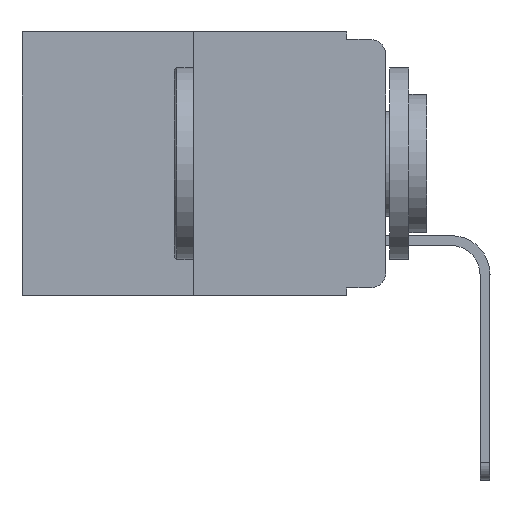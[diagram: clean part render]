
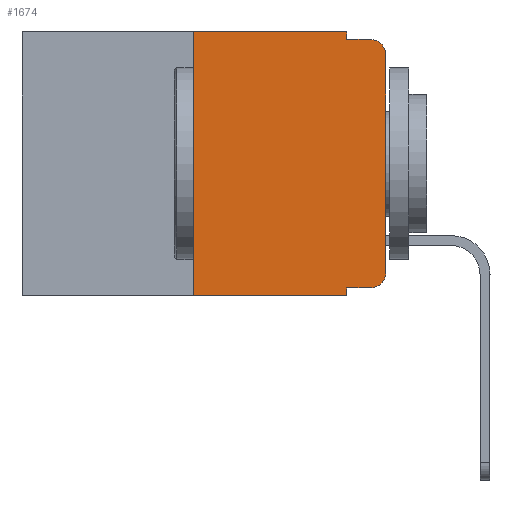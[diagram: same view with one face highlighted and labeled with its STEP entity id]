
A CAD part, left-side view. The second image highlights one B-rep face of the part: STEP entity #1674.
In plain terms, the highlighted planar face has unit normal (-1, 0, 0).
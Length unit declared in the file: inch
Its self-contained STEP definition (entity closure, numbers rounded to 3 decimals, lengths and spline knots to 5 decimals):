
#30 = LINE ( 'NONE', #6176, #9554 ) ;
#115 = VERTEX_POINT ( 'NONE', #6775 ) ;
#348 = DIRECTION ( 'NONE',  ( 0., 0., -1. ) ) ;
#703 = DIRECTION ( 'NONE',  ( 1., 0., 0. ) ) ;
#757 = VECTOR ( 'NONE', #9852, 39.37008 ) ;
#905 = EDGE_CURVE ( 'NONE', #6582, #11496, #3817, .T. ) ;
#1418 = LINE ( 'NONE', #9605, #4069 ) ;
#1454 = CARTESIAN_POINT ( 'NONE',  ( 0., 0., 0. ) ) ;
#1549 = ORIENTED_EDGE ( 'NONE', *, *, #5452, .T. ) ;
#1674 = ADVANCED_FACE ( 'NONE', ( #9595 ), #4246, .F. ) ;
#1706 = DIRECTION ( 'NONE',  ( 0., 0., 1. ) ) ;
#1743 = CARTESIAN_POINT ( 'NONE',  ( 0., 0.25, 0. ) ) ;
#1867 = VECTOR ( 'NONE', #6703, 39.37008 ) ;
#1996 = ORIENTED_EDGE ( 'NONE', *, *, #905, .F. ) ;
#2010 = CIRCLE ( 'NONE', #9799, 0.02 ) ;
#2052 = CARTESIAN_POINT ( 'NONE',  ( 0., 0.02, -0.313 ) ) ;
#2096 = LINE ( 'NONE', #9301, #5135 ) ;
#2180 = CARTESIAN_POINT ( 'NONE',  ( 0., 0.051, -0.01 ) ) ;
#2213 = DIRECTION ( 'NONE',  ( 0., -1., 0. ) ) ;
#2321 = ORIENTED_EDGE ( 'NONE', *, *, #10936, .T. ) ;
#2411 = VERTEX_POINT ( 'NONE', #9556 ) ;
#2516 = CARTESIAN_POINT ( 'NONE',  ( 0., 0.051, 0. ) ) ;
#2579 = AXIS2_PLACEMENT_3D ( 'NONE', #10174, #8378, #4041 ) ;
#2709 = DIRECTION ( 'NONE',  ( 0., -1., 0. ) ) ;
#2853 = VECTOR ( 'NONE', #9099, 39.37008 ) ;
#2990 = CARTESIAN_POINT ( 'NONE',  ( 0., 0.02, -0.333 ) ) ;
#3325 = ORIENTED_EDGE ( 'NONE', *, *, #10049, .T. ) ;
#3437 = CARTESIAN_POINT ( 'NONE',  ( 0., 0., -0.313 ) ) ;
#3559 = LINE ( 'NONE', #3613, #757 ) ;
#3613 = CARTESIAN_POINT ( 'NONE',  ( 0., 0.051, 0. ) ) ;
#3817 = LINE ( 'NONE', #5530, #2853 ) ;
#3937 = VECTOR ( 'NONE', #2709, 39.37008 ) ;
#4041 = DIRECTION ( 'NONE',  ( 0., 0., -1. ) ) ;
#4069 = VECTOR ( 'NONE', #5091, 39.37008 ) ;
#4124 = ORIENTED_EDGE ( 'NONE', *, *, #9107, .F. ) ;
#4174 = CARTESIAN_POINT ( 'NONE',  ( 0., 0.25, -0.343 ) ) ;
#4246 = PLANE ( 'NONE',  #5013 ) ;
#4949 = VERTEX_POINT ( 'NONE', #9428 ) ;
#5013 = AXIS2_PLACEMENT_3D ( 'NONE', #5121, #703, #6805 ) ;
#5091 = DIRECTION ( 'NONE',  ( 0., -1., 0. ) ) ;
#5121 = CARTESIAN_POINT ( 'NONE',  ( 0., 0.473, 0. ) ) ;
#5135 = VECTOR ( 'NONE', #2213, 39.37008 ) ;
#5156 = ORIENTED_EDGE ( 'NONE', *, *, #6040, .F. ) ;
#5393 = ORIENTED_EDGE ( 'NONE', *, *, #9227, .T. ) ;
#5452 = EDGE_CURVE ( 'NONE', #7818, #2411, #2096, .T. ) ;
#5530 = CARTESIAN_POINT ( 'NONE',  ( 0., 0.051, 0. ) ) ;
#5874 = VECTOR ( 'NONE', #1706, 39.37008 ) ;
#6040 = EDGE_CURVE ( 'NONE', #11496, #8912, #30, .T. ) ;
#6176 = CARTESIAN_POINT ( 'NONE',  ( 0., 0.051, -0.01 ) ) ;
#6582 = VERTEX_POINT ( 'NONE', #2516 ) ;
#6680 = LINE ( 'NONE', #9794, #3937 ) ;
#6703 = DIRECTION ( 'NONE',  ( 0., 0., 1. ) ) ;
#6775 = CARTESIAN_POINT ( 'NONE',  ( 0., 0.051, -0.333 ) ) ;
#6805 = DIRECTION ( 'NONE',  ( 0., 0., -1. ) ) ;
#7450 = DIRECTION ( 'NONE',  ( -1., 0., 0. ) ) ;
#7818 = VERTEX_POINT ( 'NONE', #4174 ) ;
#8344 = LINE ( 'NONE', #1743, #5874 ) ;
#8378 = DIRECTION ( 'NONE',  ( -1., 0., 0. ) ) ;
#8449 = CARTESIAN_POINT ( 'NONE',  ( 0., 0.02, -0.01 ) ) ;
#8583 = EDGE_LOOP ( 'NONE', ( #9252, #2321, #5156, #1996, #9936, #9468, #1549, #4124, #3325, #5393 ) ) ;
#8822 = DIRECTION ( 'NONE',  ( 0., -1., 0. ) ) ;
#8912 = VERTEX_POINT ( 'NONE', #8449 ) ;
#9099 = DIRECTION ( 'NONE',  ( 0., 0., -1. ) ) ;
#9107 = EDGE_CURVE ( 'NONE', #115, #2411, #3559, .T. ) ;
#9227 = EDGE_CURVE ( 'NONE', #9239, #11197, #2010, .T. ) ;
#9239 = VERTEX_POINT ( 'NONE', #2990 ) ;
#9252 = ORIENTED_EDGE ( 'NONE', *, *, #9474, .T. ) ;
#9301 = CARTESIAN_POINT ( 'NONE',  ( 0., 0.473, -0.343 ) ) ;
#9428 = CARTESIAN_POINT ( 'NONE',  ( 0., 0.25, 0. ) ) ;
#9468 = ORIENTED_EDGE ( 'NONE', *, *, #9492, .F. ) ;
#9474 = EDGE_CURVE ( 'NONE', #11197, #11133, #9878, .T. ) ;
#9492 = EDGE_CURVE ( 'NONE', #7818, #4949, #8344, .T. ) ;
#9554 = VECTOR ( 'NONE', #8822, 39.37008 ) ;
#9556 = CARTESIAN_POINT ( 'NONE',  ( 0., 0.051, -0.343 ) ) ;
#9595 = FACE_OUTER_BOUND ( 'NONE', #8583, .T. ) ;
#9605 = CARTESIAN_POINT ( 'NONE',  ( 0., 0.051, -0.333 ) ) ;
#9794 = CARTESIAN_POINT ( 'NONE',  ( 0., 0.473, 0. ) ) ;
#9799 = AXIS2_PLACEMENT_3D ( 'NONE', #2052, #7450, #348 ) ;
#9852 = DIRECTION ( 'NONE',  ( 0., 0., -1. ) ) ;
#9878 = LINE ( 'NONE', #1454, #1867 ) ;
#9936 = ORIENTED_EDGE ( 'NONE', *, *, #10733, .F. ) ;
#10049 = EDGE_CURVE ( 'NONE', #115, #9239, #1418, .T. ) ;
#10174 = CARTESIAN_POINT ( 'NONE',  ( 0., 0.02, -0.03 ) ) ;
#10733 = EDGE_CURVE ( 'NONE', #4949, #6582, #6680, .T. ) ;
#10936 = EDGE_CURVE ( 'NONE', #11133, #8912, #11287, .T. ) ;
#11133 = VERTEX_POINT ( 'NONE', #11253 ) ;
#11197 = VERTEX_POINT ( 'NONE', #3437 ) ;
#11253 = CARTESIAN_POINT ( 'NONE',  ( 0., 0., -0.03 ) ) ;
#11287 = CIRCLE ( 'NONE', #2579, 0.02 ) ;
#11496 = VERTEX_POINT ( 'NONE', #2180 ) ;
